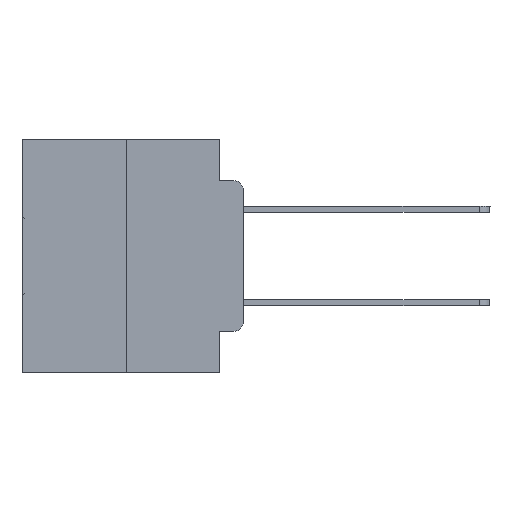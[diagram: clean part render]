
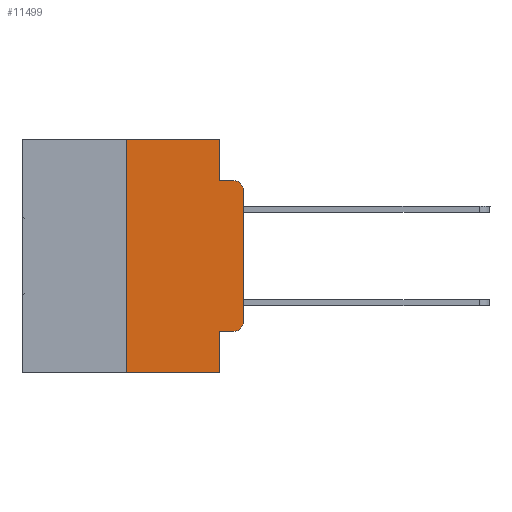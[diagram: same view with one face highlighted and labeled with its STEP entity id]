
A CAD part, left-side view. The second image highlights one B-rep face of the part: STEP entity #11499.
In plain terms, the highlighted planar face has unit normal (-1, 0, 0).
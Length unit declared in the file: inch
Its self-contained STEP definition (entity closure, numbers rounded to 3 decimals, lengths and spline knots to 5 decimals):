
#418 = DIRECTION ( 'NONE',  ( 0., 0., 1. ) ) ;
#659 = DIRECTION ( 'NONE',  ( 0., 0., -1. ) ) ;
#682 = DIRECTION ( 'NONE',  ( 0., -1., 0. ) ) ;
#1830 = ORIENTED_EDGE ( 'NONE', *, *, #23950, .T. ) ;
#2591 = CARTESIAN_POINT ( 'NONE',  ( 0., 0.25, 0. ) ) ;
#2900 = FACE_OUTER_BOUND ( 'NONE', #19307, .T. ) ;
#3186 = ORIENTED_EDGE ( 'NONE', *, *, #32347, .T. ) ;
#3999 = AXIS2_PLACEMENT_3D ( 'NONE', #13306, #13136, #8601 ) ;
#5009 = ORIENTED_EDGE ( 'NONE', *, *, #30166, .F. ) ;
#5117 = CIRCLE ( 'NONE', #11580, 0.02 ) ;
#5129 = LINE ( 'NONE', #23392, #31524 ) ;
#5230 = VERTEX_POINT ( 'NONE', #21224 ) ;
#5598 = DIRECTION ( 'NONE',  ( 0., -1., 0. ) ) ;
#5719 = VECTOR ( 'NONE', #31856, 39.37008 ) ;
#6814 = AXIS2_PLACEMENT_3D ( 'NONE', #17232, #9859, #24930 ) ;
#7232 = LINE ( 'NONE', #17444, #19592 ) ;
#7355 = CIRCLE ( 'NONE', #6814, 0.02 ) ;
#8464 = CARTESIAN_POINT ( 'NONE',  ( 0., 0.051, -0.4115 ) ) ;
#8601 = DIRECTION ( 'NONE',  ( 0., 0., -1. ) ) ;
#8702 = EDGE_CURVE ( 'NONE', #29319, #32658, #17683, .T. ) ;
#9065 = VERTEX_POINT ( 'NONE', #31576 ) ;
#9157 = EDGE_CURVE ( 'NONE', #32658, #28502, #7232, .T. ) ;
#9405 = ORIENTED_EDGE ( 'NONE', *, *, #21501, .F. ) ;
#9421 = CARTESIAN_POINT ( 'NONE',  ( 0., 0.02, -0.0885 ) ) ;
#9859 = DIRECTION ( 'NONE',  ( -1., 0., 0. ) ) ;
#10156 = CARTESIAN_POINT ( 'NONE',  ( 0., 0.02, -0.1085 ) ) ;
#11499 = ADVANCED_FACE ( 'NONE', ( #2900 ), #31587, .F. ) ;
#11548 = CARTESIAN_POINT ( 'NONE',  ( 0., 0.25, -0.5 ) ) ;
#11580 = AXIS2_PLACEMENT_3D ( 'NONE', #10156, #20359, #30625 ) ;
#11731 = EDGE_CURVE ( 'NONE', #25226, #9065, #14785, .T. ) ;
#12417 = DIRECTION ( 'NONE',  ( 0., -1., 0. ) ) ;
#12759 = LINE ( 'NONE', #22961, #25015 ) ;
#13136 = DIRECTION ( 'NONE',  ( 1., 0., 0. ) ) ;
#13306 = CARTESIAN_POINT ( 'NONE',  ( 0., 0.473, 0. ) ) ;
#13755 = VERTEX_POINT ( 'NONE', #18549 ) ;
#13845 = ORIENTED_EDGE ( 'NONE', *, *, #21119, .T. ) ;
#14785 = LINE ( 'NONE', #17297, #16380 ) ;
#15172 = DIRECTION ( 'NONE',  ( 0., 0., 1. ) ) ;
#15375 = VERTEX_POINT ( 'NONE', #25237 ) ;
#15957 = LINE ( 'NONE', #26668, #18564 ) ;
#16380 = VECTOR ( 'NONE', #33052, 39.37008 ) ;
#17232 = CARTESIAN_POINT ( 'NONE',  ( 0., 0.02, -0.3915 ) ) ;
#17297 = CARTESIAN_POINT ( 'NONE',  ( 0., 0.051, 0. ) ) ;
#17444 = CARTESIAN_POINT ( 'NONE',  ( 0., 0.473, 0. ) ) ;
#17504 = CARTESIAN_POINT ( 'NONE',  ( 0., 0.25, 0. ) ) ;
#17683 = LINE ( 'NONE', #2591, #21185 ) ;
#17962 = ORIENTED_EDGE ( 'NONE', *, *, #11731, .F. ) ;
#18549 = CARTESIAN_POINT ( 'NONE',  ( 0., 0.051, -0.0885 ) ) ;
#18564 = VECTOR ( 'NONE', #682, 39.37008 ) ;
#18704 = VERTEX_POINT ( 'NONE', #9421 ) ;
#19307 = EDGE_LOOP ( 'NONE', ( #3186, #13845, #9405, #5009, #23594, #21547, #1830, #17962, #21651, #28935 ) ) ;
#19592 = VECTOR ( 'NONE', #12417, 39.37008 ) ;
#19874 = EDGE_CURVE ( 'NONE', #25226, #15375, #20858, .T. ) ;
#20359 = DIRECTION ( 'NONE',  ( -1., 0., 0. ) ) ;
#20858 = LINE ( 'NONE', #8464, #27560 ) ;
#21119 = EDGE_CURVE ( 'NONE', #27752, #18704, #5117, .T. ) ;
#21185 = VECTOR ( 'NONE', #15172, 39.37008 ) ;
#21224 = CARTESIAN_POINT ( 'NONE',  ( 0., 0., -0.3915 ) ) ;
#21501 = EDGE_CURVE ( 'NONE', #13755, #18704, #15957, .T. ) ;
#21547 = ORIENTED_EDGE ( 'NONE', *, *, #8702, .F. ) ;
#21651 = ORIENTED_EDGE ( 'NONE', *, *, #19874, .T. ) ;
#21934 = CARTESIAN_POINT ( 'NONE',  ( 0., 0.473, -0.5 ) ) ;
#22961 = CARTESIAN_POINT ( 'NONE',  ( 0., 0.051, 0. ) ) ;
#22971 = CARTESIAN_POINT ( 'NONE',  ( 0., 0.051, 0. ) ) ;
#23392 = CARTESIAN_POINT ( 'NONE',  ( 0., 0., 0. ) ) ;
#23594 = ORIENTED_EDGE ( 'NONE', *, *, #9157, .F. ) ;
#23950 = EDGE_CURVE ( 'NONE', #29319, #9065, #26629, .T. ) ;
#24120 = EDGE_CURVE ( 'NONE', #15375, #5230, #7355, .T. ) ;
#24366 = CARTESIAN_POINT ( 'NONE',  ( 0., 0., -0.1085 ) ) ;
#24930 = DIRECTION ( 'NONE',  ( 0., 0., -1. ) ) ;
#25015 = VECTOR ( 'NONE', #659, 39.37008 ) ;
#25226 = VERTEX_POINT ( 'NONE', #26498 ) ;
#25237 = CARTESIAN_POINT ( 'NONE',  ( 0., 0.02, -0.4115 ) ) ;
#26498 = CARTESIAN_POINT ( 'NONE',  ( 0., 0.051, -0.4115 ) ) ;
#26629 = LINE ( 'NONE', #21934, #5719 ) ;
#26668 = CARTESIAN_POINT ( 'NONE',  ( 0., 0.051, -0.0885 ) ) ;
#27560 = VECTOR ( 'NONE', #5598, 39.37008 ) ;
#27752 = VERTEX_POINT ( 'NONE', #24366 ) ;
#28502 = VERTEX_POINT ( 'NONE', #22971 ) ;
#28935 = ORIENTED_EDGE ( 'NONE', *, *, #24120, .T. ) ;
#29319 = VERTEX_POINT ( 'NONE', #11548 ) ;
#30166 = EDGE_CURVE ( 'NONE', #28502, #13755, #12759, .T. ) ;
#30625 = DIRECTION ( 'NONE',  ( 0., 0., -1. ) ) ;
#31524 = VECTOR ( 'NONE', #418, 39.37008 ) ;
#31576 = CARTESIAN_POINT ( 'NONE',  ( 0., 0.051, -0.5 ) ) ;
#31587 = PLANE ( 'NONE',  #3999 ) ;
#31856 = DIRECTION ( 'NONE',  ( 0., -1., 0. ) ) ;
#32347 = EDGE_CURVE ( 'NONE', #5230, #27752, #5129, .T. ) ;
#32658 = VERTEX_POINT ( 'NONE', #17504 ) ;
#33052 = DIRECTION ( 'NONE',  ( 0., 0., -1. ) ) ;
